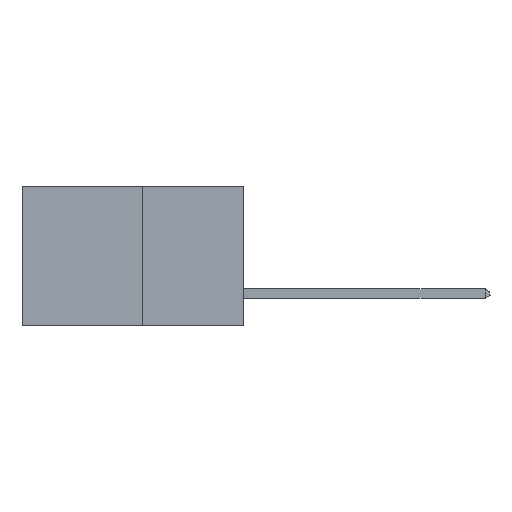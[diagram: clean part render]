
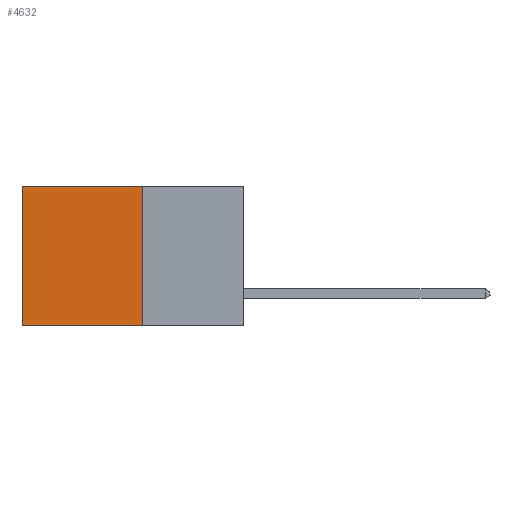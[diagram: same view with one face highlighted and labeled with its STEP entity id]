
A CAD part, left-side view. The second image highlights one B-rep face of the part: STEP entity #4632.
In plain terms, the highlighted planar face has unit normal (-1, 0, 0).
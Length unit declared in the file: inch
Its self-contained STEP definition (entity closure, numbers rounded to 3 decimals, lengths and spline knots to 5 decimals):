
#308 = CARTESIAN_POINT ( 'NONE',  ( 0.277, 0.27, -0.37 ) ) ;
#1657 = VECTOR ( 'NONE', #5704, 39.37008 ) ;
#3169 = CARTESIAN_POINT ( 'NONE',  ( 0.277, 0.59, -0.37 ) ) ;
#3485 = CARTESIAN_POINT ( 'NONE',  ( 0.277, 0.59, -0.37 ) ) ;
#4318 = AXIS2_PLACEMENT_3D ( 'NONE', #6789, #6597, #6210 ) ;
#4632 = ADVANCED_FACE ( 'NONE', ( #21002 ), #7738, .F. ) ;
#5260 = VERTEX_POINT ( 'NONE', #3485 ) ;
#5460 = VECTOR ( 'NONE', #27262, 39.37008 ) ;
#5474 = ORIENTED_EDGE ( 'NONE', *, *, #24389, .F. ) ;
#5704 = DIRECTION ( 'NONE',  ( 0., 1., 0. ) ) ;
#6210 = DIRECTION ( 'NONE',  ( 0., 0., -1. ) ) ;
#6597 = DIRECTION ( 'NONE',  ( 1., 0., 0. ) ) ;
#6789 = CARTESIAN_POINT ( 'NONE',  ( 0.277, 0.27, -0.37 ) ) ;
#6988 = VECTOR ( 'NONE', #25871, 39.37008 ) ;
#7257 = ORIENTED_EDGE ( 'NONE', *, *, #19044, .T. ) ;
#7738 = PLANE ( 'NONE',  #4318 ) ;
#8568 = CARTESIAN_POINT ( 'NONE',  ( 0.277, 0.59, 0. ) ) ;
#10145 = VERTEX_POINT ( 'NONE', #8568 ) ;
#10710 = EDGE_CURVE ( 'NONE', #21805, #10145, #13598, .T. ) ;
#11358 = CARTESIAN_POINT ( 'NONE',  ( 0.277, 0.27, 0. ) ) ;
#12019 = CARTESIAN_POINT ( 'NONE',  ( 0.277, 0.27, 0. ) ) ;
#13598 = LINE ( 'NONE', #11358, #19694 ) ;
#13712 = LINE ( 'NONE', #3169, #6988 ) ;
#14776 = ORIENTED_EDGE ( 'NONE', *, *, #20410, .F. ) ;
#16988 = CARTESIAN_POINT ( 'NONE',  ( 0.277, 0.27, -0.37 ) ) ;
#18371 = ORIENTED_EDGE ( 'NONE', *, *, #10710, .T. ) ;
#19044 = EDGE_CURVE ( 'NONE', #10145, #5260, #13712, .T. ) ;
#19694 = VECTOR ( 'NONE', #27320, 39.37008 ) ;
#20410 = EDGE_CURVE ( 'NONE', #21805, #23579, #23627, .T. ) ;
#20508 = EDGE_LOOP ( 'NONE', ( #7257, #5474, #14776, #18371 ) ) ;
#21002 = FACE_OUTER_BOUND ( 'NONE', #20508, .T. ) ;
#21296 = LINE ( 'NONE', #16988, #1657 ) ;
#21805 = VERTEX_POINT ( 'NONE', #12019 ) ;
#22714 = CARTESIAN_POINT ( 'NONE',  ( 0.277, 0.27, -0.37 ) ) ;
#23579 = VERTEX_POINT ( 'NONE', #308 ) ;
#23627 = LINE ( 'NONE', #22714, #5460 ) ;
#24389 = EDGE_CURVE ( 'NONE', #23579, #5260, #21296, .T. ) ;
#25871 = DIRECTION ( 'NONE',  ( 0., 0., -1. ) ) ;
#27262 = DIRECTION ( 'NONE',  ( 0., 0., -1. ) ) ;
#27320 = DIRECTION ( 'NONE',  ( 0., 1., 0. ) ) ;
